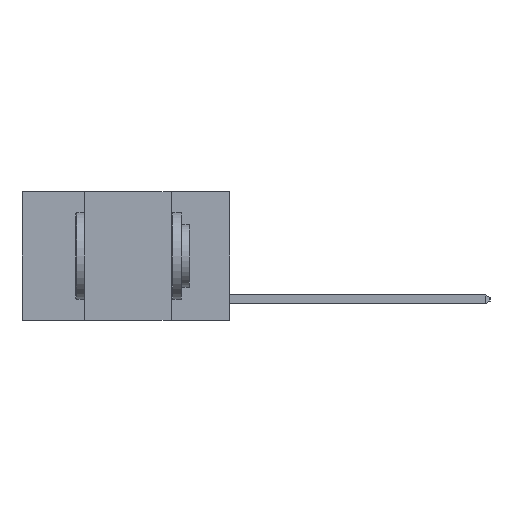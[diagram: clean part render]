
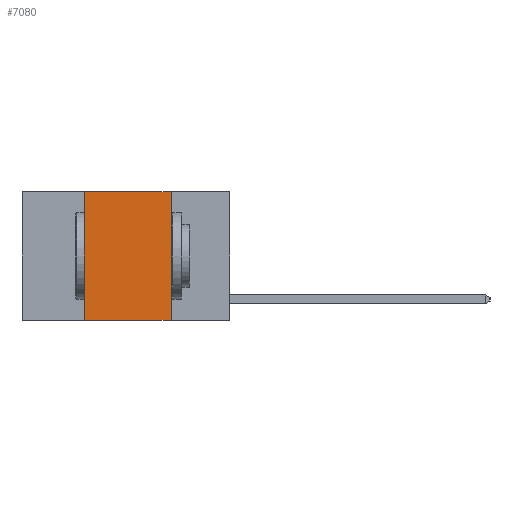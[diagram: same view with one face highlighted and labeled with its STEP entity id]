
A CAD part, left-side view. The second image highlights one B-rep face of the part: STEP entity #7080.
In plain terms, the highlighted planar face has unit normal (-1, 0, 0).
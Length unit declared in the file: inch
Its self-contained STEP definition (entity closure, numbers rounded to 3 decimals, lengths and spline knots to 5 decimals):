
#55 = EDGE_CURVE ( 'NONE', #838, #1361, #8387, .T. ) ;
#243 = VECTOR ( 'NONE', #3803, 39.37008 ) ;
#383 = AXIS2_PLACEMENT_3D ( 'NONE', #7094, #7823, #3276 ) ;
#838 = VERTEX_POINT ( 'NONE', #8058 ) ;
#864 = CARTESIAN_POINT ( 'NONE',  ( 0., 0.17, 0. ) ) ;
#1361 = VERTEX_POINT ( 'NONE', #7520 ) ;
#1424 = CARTESIAN_POINT ( 'NONE',  ( 0., 0.42, 0. ) ) ;
#1956 = DIRECTION ( 'NONE',  ( 0., 0., -1. ) ) ;
#2043 = FACE_OUTER_BOUND ( 'NONE', #4403, .T. ) ;
#2353 = LINE ( 'NONE', #1424, #243 ) ;
#2366 = VERTEX_POINT ( 'NONE', #864 ) ;
#2448 = PLANE ( 'NONE',  #383 ) ;
#2932 = DIRECTION ( 'NONE',  ( 0., -1., 0. ) ) ;
#2963 = VERTEX_POINT ( 'NONE', #4051 ) ;
#3020 = ORIENTED_EDGE ( 'NONE', *, *, #5510, .F. ) ;
#3276 = DIRECTION ( 'NONE',  ( 0., 0., -1. ) ) ;
#3621 = ORIENTED_EDGE ( 'NONE', *, *, #9596, .F. ) ;
#3803 = DIRECTION ( 'NONE',  ( 0., 0., 1. ) ) ;
#4051 = CARTESIAN_POINT ( 'NONE',  ( 0., 0.42, 0. ) ) ;
#4403 = EDGE_LOOP ( 'NONE', ( #3020, #3621, #7011, #9060 ) ) ;
#4483 = EDGE_CURVE ( 'NONE', #838, #2963, #2353, .T. ) ;
#4769 = LINE ( 'NONE', #7353, #6799 ) ;
#5510 = EDGE_CURVE ( 'NONE', #2366, #1361, #4769, .T. ) ;
#5755 = VECTOR ( 'NONE', #2932, 39.37008 ) ;
#6799 = VECTOR ( 'NONE', #1956, 39.37008 ) ;
#7011 = ORIENTED_EDGE ( 'NONE', *, *, #4483, .F. ) ;
#7080 = ADVANCED_FACE ( 'NONE', ( #2043 ), #2448, .F. ) ;
#7094 = CARTESIAN_POINT ( 'NONE',  ( 0., 0.6, 0. ) ) ;
#7353 = CARTESIAN_POINT ( 'NONE',  ( 0., 0.17, 0. ) ) ;
#7507 = CARTESIAN_POINT ( 'NONE',  ( 0., 0.6, 0. ) ) ;
#7520 = CARTESIAN_POINT ( 'NONE',  ( 0., 0.17, -0.37 ) ) ;
#7823 = DIRECTION ( 'NONE',  ( 1., 0., 0. ) ) ;
#7986 = LINE ( 'NONE', #7507, #5755 ) ;
#8058 = CARTESIAN_POINT ( 'NONE',  ( 0., 0.42, -0.37 ) ) ;
#8387 = LINE ( 'NONE', #8411, #8616 ) ;
#8411 = CARTESIAN_POINT ( 'NONE',  ( 0., 0.6, -0.37 ) ) ;
#8616 = VECTOR ( 'NONE', #9159, 39.37008 ) ;
#9060 = ORIENTED_EDGE ( 'NONE', *, *, #55, .T. ) ;
#9159 = DIRECTION ( 'NONE',  ( 0., -1., 0. ) ) ;
#9596 = EDGE_CURVE ( 'NONE', #2963, #2366, #7986, .T. ) ;
